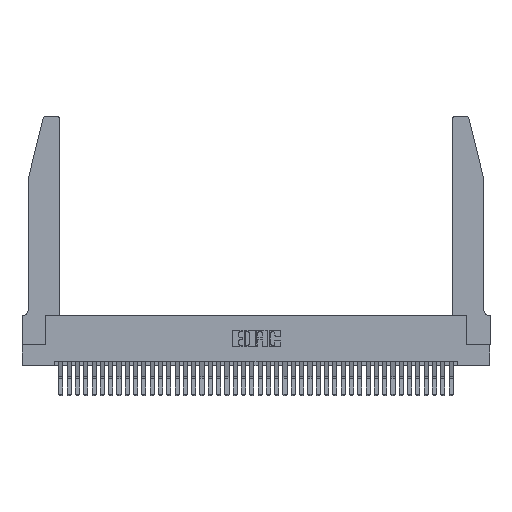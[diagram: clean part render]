
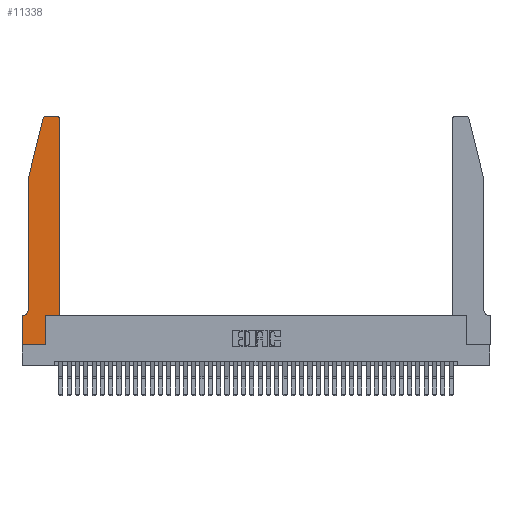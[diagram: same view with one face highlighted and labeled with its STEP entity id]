
A CAD part, top view. The second image highlights one B-rep face of the part: STEP entity #11338.
In plain terms, the highlighted planar face has unit normal (0, 0, 1).
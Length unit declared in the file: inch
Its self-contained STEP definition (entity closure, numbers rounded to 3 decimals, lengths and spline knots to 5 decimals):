
#822 = CARTESIAN_POINT ( 'NONE',  ( 0., 0.35, 0.37 ) ) ;
#1830 = CARTESIAN_POINT ( 'NONE',  ( 0.4505, 0.35, 0.37 ) ) ;
#1967 = ORIENTED_EDGE ( 'NONE', *, *, #37362, .T. ) ;
#2124 = LINE ( 'NONE', #1830, #31304 ) ;
#2401 = LINE ( 'NONE', #16412, #35628 ) ;
#2429 = DIRECTION ( 'NONE',  ( -1., 0., 0. ) ) ;
#2555 = VECTOR ( 'NONE', #18857, 39.37008 ) ;
#2707 = VERTEX_POINT ( 'NONE', #20835 ) ;
#2902 = CARTESIAN_POINT ( 'NONE',  ( 0.4505, 0.35, 0.37 ) ) ;
#3014 = CARTESIAN_POINT ( 'NONE',  ( 0.4505, 2.72, 0.37 ) ) ;
#3981 = EDGE_CURVE ( 'NONE', #9924, #32779, #36537, .T. ) ;
#4083 = DIRECTION ( 'NONE',  ( 0., 0., 1. ) ) ;
#5833 = LINE ( 'NONE', #20540, #26395 ) ;
#6890 = VECTOR ( 'NONE', #11423, 39.37008 ) ;
#7873 = VECTOR ( 'NONE', #39524, 39.37008 ) ;
#8140 = VERTEX_POINT ( 'NONE', #26785 ) ;
#8801 = VECTOR ( 'NONE', #12911, 39.37008 ) ;
#9415 = AXIS2_PLACEMENT_3D ( 'NONE', #32585, #38777, #35938 ) ;
#9599 = ORIENTED_EDGE ( 'NONE', *, *, #26160, .T. ) ;
#9924 = VERTEX_POINT ( 'NONE', #34903 ) ;
#10061 = LINE ( 'NONE', #32110, #27157 ) ;
#10237 = CARTESIAN_POINT ( 'NONE',  ( 0.0055, 0.35, 0.37 ) ) ;
#11171 = FACE_OUTER_BOUND ( 'NONE', #15019, .T. ) ;
#11338 = ADVANCED_FACE ( 'NONE', ( #11171 ), #36147, .T. ) ;
#11423 = DIRECTION ( 'NONE',  ( 0., -1., 0. ) ) ;
#11477 = VERTEX_POINT ( 'NONE', #3014 ) ;
#11537 = VERTEX_POINT ( 'NONE', #10237 ) ;
#12145 = EDGE_CURVE ( 'NONE', #37016, #9924, #30264, .T. ) ;
#12911 = DIRECTION ( 'NONE',  ( 0., 1., 0. ) ) ;
#14023 = CARTESIAN_POINT ( 'NONE',  ( 0.284, 2.72, 0.37 ) ) ;
#14371 = DIRECTION ( 'NONE',  ( 1., 0., 0. ) ) ;
#14984 = EDGE_CURVE ( 'NONE', #20770, #17329, #5833, .T. ) ;
#15019 = EDGE_LOOP ( 'NONE', ( #36001, #9599, #32875, #23086, #24410, #27788, #25109, #26900, #40241, #21759, #24104, #1967 ) ) ;
#15223 = CARTESIAN_POINT ( 'NONE',  ( 0.0055, 0.42, 0.37 ) ) ;
#15513 = CARTESIAN_POINT ( 'NONE',  ( 0.25487, 2.72718, 0.37 ) ) ;
#16048 = DIRECTION ( 'NONE',  ( -1., 0., 0. ) ) ;
#16412 = CARTESIAN_POINT ( 'NONE',  ( 0.2605, 2.75, 0.37 ) ) ;
#16919 = EDGE_CURVE ( 'NONE', #18142, #28158, #2124, .T. ) ;
#17273 = LINE ( 'NONE', #2902, #8801 ) ;
#17329 = VERTEX_POINT ( 'NONE', #36201 ) ;
#17510 = CARTESIAN_POINT ( 'NONE',  ( 0.2865, 0.35, 0.37 ) ) ;
#18142 = VERTEX_POINT ( 'NONE', #34467 ) ;
#18857 = DIRECTION ( 'NONE',  ( -0.239, -0.971, 0. ) ) ;
#18995 = CARTESIAN_POINT ( 'NONE',  ( 0.0755, 2., 0.37 ) ) ;
#20540 = CARTESIAN_POINT ( 'NONE',  ( 0., 0., 0.37 ) ) ;
#20770 = VERTEX_POINT ( 'NONE', #28853 ) ;
#20835 = CARTESIAN_POINT ( 'NONE',  ( 0.284, 2.75, 0.37 ) ) ;
#20918 = AXIS2_PLACEMENT_3D ( 'NONE', #15223, #25252, #2429 ) ;
#21759 = ORIENTED_EDGE ( 'NONE', *, *, #16919, .T. ) ;
#21976 = LINE ( 'NONE', #33349, #7873 ) ;
#23086 = ORIENTED_EDGE ( 'NONE', *, *, #3981, .T. ) ;
#23530 = DIRECTION ( 'NONE',  ( 1., 0., 0. ) ) ;
#23786 = AXIS2_PLACEMENT_3D ( 'NONE', #822, #4083, #23530 ) ;
#24088 = DIRECTION ( 'NONE',  ( 0., -1., 0. ) ) ;
#24104 = ORIENTED_EDGE ( 'NONE', *, *, #28152, .T. ) ;
#24410 = ORIENTED_EDGE ( 'NONE', *, *, #35986, .T. ) ;
#24571 = AXIS2_PLACEMENT_3D ( 'NONE', #14023, #33722, #34011 ) ;
#25109 = ORIENTED_EDGE ( 'NONE', *, *, #14984, .T. ) ;
#25252 = DIRECTION ( 'NONE',  ( 0., 0., -1. ) ) ;
#26160 = EDGE_CURVE ( 'NONE', #2707, #37016, #28088, .T. ) ;
#26395 = VECTOR ( 'NONE', #24088, 39.37008 ) ;
#26523 = EDGE_CURVE ( 'NONE', #17329, #8140, #21976, .T. ) ;
#26785 = CARTESIAN_POINT ( 'NONE',  ( 0.2865, 0., 0.37 ) ) ;
#26900 = ORIENTED_EDGE ( 'NONE', *, *, #26523, .T. ) ;
#27157 = VECTOR ( 'NONE', #16048, 39.37008 ) ;
#27312 = CARTESIAN_POINT ( 'NONE',  ( 0.0755, 2., 0.37 ) ) ;
#27788 = ORIENTED_EDGE ( 'NONE', *, *, #32681, .T. ) ;
#28088 = CIRCLE ( 'NONE', #24571, 0.03 ) ;
#28152 = EDGE_CURVE ( 'NONE', #28158, #11477, #17273, .T. ) ;
#28158 = VERTEX_POINT ( 'NONE', #38227 ) ;
#28853 = CARTESIAN_POINT ( 'NONE',  ( 0., 0.35, 0.37 ) ) ;
#29277 = DIRECTION ( 'NONE',  ( -1., 0., 0. ) ) ;
#30264 = LINE ( 'NONE', #18995, #2555 ) ;
#30854 = LINE ( 'NONE', #17510, #35383 ) ;
#31105 = EDGE_CURVE ( 'NONE', #8140, #18142, #30854, .T. ) ;
#31304 = VECTOR ( 'NONE', #14371, 39.37008 ) ;
#32049 = CIRCLE ( 'NONE', #20918, 0.07 ) ;
#32110 = CARTESIAN_POINT ( 'NONE',  ( 0.0755, 0.35, 0.37 ) ) ;
#32585 = CARTESIAN_POINT ( 'NONE',  ( 0.4205, 2.72, 0.37 ) ) ;
#32681 = EDGE_CURVE ( 'NONE', #11537, #20770, #10061, .T. ) ;
#32779 = VERTEX_POINT ( 'NONE', #33053 ) ;
#32875 = ORIENTED_EDGE ( 'NONE', *, *, #12145, .T. ) ;
#33053 = CARTESIAN_POINT ( 'NONE',  ( 0.0755, 0.42, 0.37 ) ) ;
#33346 = VERTEX_POINT ( 'NONE', #35557 ) ;
#33349 = CARTESIAN_POINT ( 'NONE',  ( 0., 0., 0.37 ) ) ;
#33363 = CIRCLE ( 'NONE', #9415, 0.03 ) ;
#33722 = DIRECTION ( 'NONE',  ( 0., 0., 1. ) ) ;
#34011 = DIRECTION ( 'NONE',  ( 1., 0., 0. ) ) ;
#34467 = CARTESIAN_POINT ( 'NONE',  ( 0.2865, 0.35, 0.37 ) ) ;
#34903 = CARTESIAN_POINT ( 'NONE',  ( 0.0755, 2., 0.37 ) ) ;
#35383 = VECTOR ( 'NONE', #37360, 39.37008 ) ;
#35557 = CARTESIAN_POINT ( 'NONE',  ( 0.4205, 2.75, 0.37 ) ) ;
#35628 = VECTOR ( 'NONE', #29277, 39.37008 ) ;
#35938 = DIRECTION ( 'NONE',  ( 1., 0., 0. ) ) ;
#35986 = EDGE_CURVE ( 'NONE', #32779, #11537, #32049, .T. ) ;
#36001 = ORIENTED_EDGE ( 'NONE', *, *, #40953, .T. ) ;
#36147 = PLANE ( 'NONE',  #23786 ) ;
#36201 = CARTESIAN_POINT ( 'NONE',  ( 0., 0., 0.37 ) ) ;
#36537 = LINE ( 'NONE', #27312, #6890 ) ;
#37016 = VERTEX_POINT ( 'NONE', #15513 ) ;
#37360 = DIRECTION ( 'NONE',  ( 0., 1., 0. ) ) ;
#37362 = EDGE_CURVE ( 'NONE', #11477, #33346, #33363, .T. ) ;
#38227 = CARTESIAN_POINT ( 'NONE',  ( 0.4505, 0.35, 0.37 ) ) ;
#38777 = DIRECTION ( 'NONE',  ( 0., 0., 1. ) ) ;
#39524 = DIRECTION ( 'NONE',  ( 1., 0., 0. ) ) ;
#40241 = ORIENTED_EDGE ( 'NONE', *, *, #31105, .T. ) ;
#40953 = EDGE_CURVE ( 'NONE', #33346, #2707, #2401, .T. ) ;
